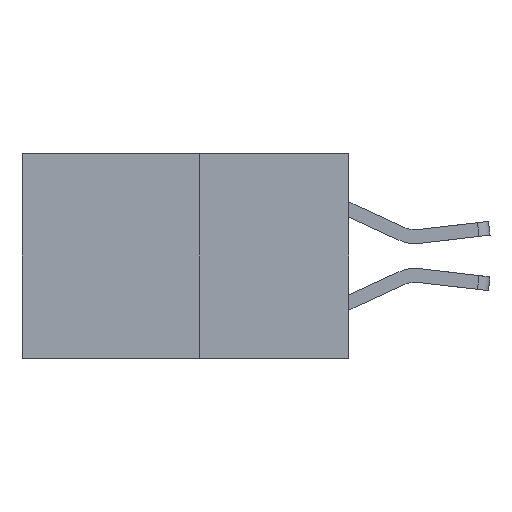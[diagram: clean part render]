
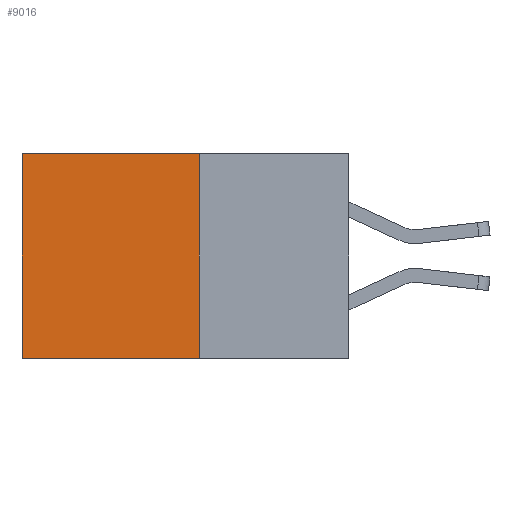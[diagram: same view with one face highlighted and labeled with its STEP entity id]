
A CAD part, left-side view. The second image highlights one B-rep face of the part: STEP entity #9016.
In plain terms, the highlighted planar face has unit normal (-1, 0, 0).
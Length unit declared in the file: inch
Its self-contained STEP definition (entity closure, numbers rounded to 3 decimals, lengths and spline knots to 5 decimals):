
#6 = LINE ( 'NONE', #8762, #5754 ) ;
#230 = DIRECTION ( 'NONE',  ( 0., 0., -1. ) ) ;
#556 = VECTOR ( 'NONE', #6511, 39.37008 ) ;
#560 = CARTESIAN_POINT ( 'NONE',  ( 0.277, 0.27, -0.37 ) ) ;
#636 = CARTESIAN_POINT ( 'NONE',  ( 0.277, 0.27, -0.37 ) ) ;
#905 = EDGE_CURVE ( 'NONE', #5452, #4714, #6, .T. ) ;
#1046 = EDGE_LOOP ( 'NONE', ( #5220, #4489, #3259, #2020 ) ) ;
#1390 = DIRECTION ( 'NONE',  ( 1., 0., 0. ) ) ;
#1515 = EDGE_CURVE ( 'NONE', #7752, #4714, #6530, .T. ) ;
#1555 = FACE_OUTER_BOUND ( 'NONE', #1046, .T. ) ;
#1681 = CARTESIAN_POINT ( 'NONE',  ( 0.277, 0.27, 0. ) ) ;
#2020 = ORIENTED_EDGE ( 'NONE', *, *, #8628, .T. ) ;
#2369 = CARTESIAN_POINT ( 'NONE',  ( 0.277, 0.59, -0.37 ) ) ;
#3259 = ORIENTED_EDGE ( 'NONE', *, *, #6824, .F. ) ;
#3884 = CARTESIAN_POINT ( 'NONE',  ( 0.277, 0.27, -0.37 ) ) ;
#3887 = DIRECTION ( 'NONE',  ( 0., 1., 0. ) ) ;
#4037 = LINE ( 'NONE', #1681, #7149 ) ;
#4489 = ORIENTED_EDGE ( 'NONE', *, *, #1515, .F. ) ;
#4714 = VERTEX_POINT ( 'NONE', #2369 ) ;
#4984 = PLANE ( 'NONE',  #7242 ) ;
#5220 = ORIENTED_EDGE ( 'NONE', *, *, #905, .T. ) ;
#5452 = VERTEX_POINT ( 'NONE', #7626 ) ;
#5754 = VECTOR ( 'NONE', #8830, 39.37008 ) ;
#5824 = CARTESIAN_POINT ( 'NONE',  ( 0.277, 0.27, 0. ) ) ;
#6404 = DIRECTION ( 'NONE',  ( 0., 0., -1. ) ) ;
#6511 = DIRECTION ( 'NONE',  ( 0., 1., 0. ) ) ;
#6530 = LINE ( 'NONE', #7870, #556 ) ;
#6824 = EDGE_CURVE ( 'NONE', #9160, #7752, #7274, .T. ) ;
#7149 = VECTOR ( 'NONE', #3887, 39.37008 ) ;
#7242 = AXIS2_PLACEMENT_3D ( 'NONE', #636, #1390, #6404 ) ;
#7274 = LINE ( 'NONE', #3884, #7728 ) ;
#7626 = CARTESIAN_POINT ( 'NONE',  ( 0.277, 0.59, 0. ) ) ;
#7728 = VECTOR ( 'NONE', #230, 39.37008 ) ;
#7752 = VERTEX_POINT ( 'NONE', #560 ) ;
#7870 = CARTESIAN_POINT ( 'NONE',  ( 0.277, 0.27, -0.37 ) ) ;
#8628 = EDGE_CURVE ( 'NONE', #9160, #5452, #4037, .T. ) ;
#8762 = CARTESIAN_POINT ( 'NONE',  ( 0.277, 0.59, -0.37 ) ) ;
#8830 = DIRECTION ( 'NONE',  ( 0., 0., -1. ) ) ;
#9016 = ADVANCED_FACE ( 'NONE', ( #1555 ), #4984, .F. ) ;
#9160 = VERTEX_POINT ( 'NONE', #5824 ) ;
